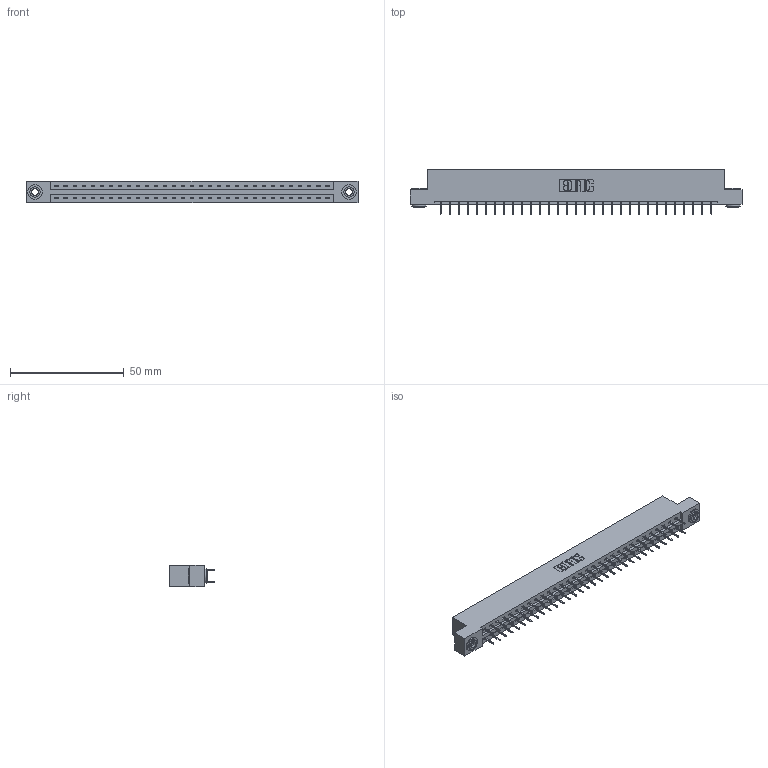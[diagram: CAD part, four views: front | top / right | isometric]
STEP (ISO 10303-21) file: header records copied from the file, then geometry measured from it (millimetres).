
FILE_DESCRIPTION (( 'STEP AP203' ), '1' );
FILE_NAME ('387-062-524-203.STEP', '2019-10-19T14:49:27', ( '' ), ( '' ), 'SwSTEP 2.0', 'SolidWorks 2016', '' );
FILE_SCHEMA (( 'CONFIG_CONTROL_DESIGN' ));
Length unit declared in the file: inch
Products named in the file (4): 345-292-001_345-293-124; 337 Part_Flush Mounting Lugs - 0.156 Dia-TH; 345-250-002_345-250-002-102; 387-062-524-203
Assembly tree (65 placements, depth 2):
  387-062-524-203
    337 Part_Flush Mounting Lugs - 0.156 Dia-TH
    345-292-001_345-293-124  x62
    345-250-002_345-250-002-102  x2
Bounding box: 145.85 x 19.69 x 9.4 mm (x, y, z)
Volume: 15149.6 mm3; surface area: 16953.7 mm2
Topology: 65 solids, 65 shells, 3748 faces, 10617 edges, 6826 vertices
Faces by surface type: plane 2808, cylinder 932, cone 8
Entity records: 26182 total; most frequent: CARTESIAN_POINT 4393, ORIENTED_EDGE 4322, DIRECTION 3791, EDGE_CURVE 2161, VECTOR 2013, LINE 2013, VERTEX_POINT 1434, AXIS2_PLACEMENT_3D 889
